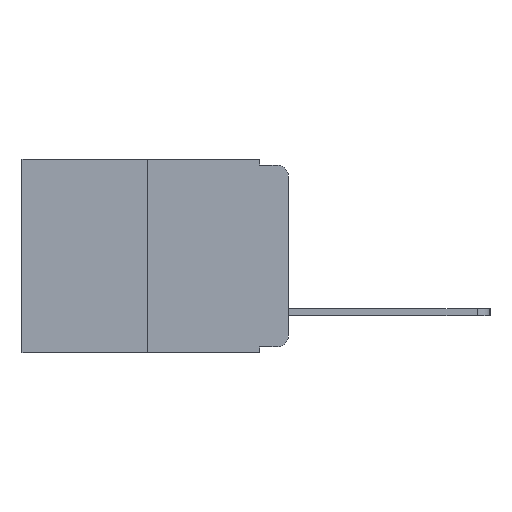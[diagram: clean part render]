
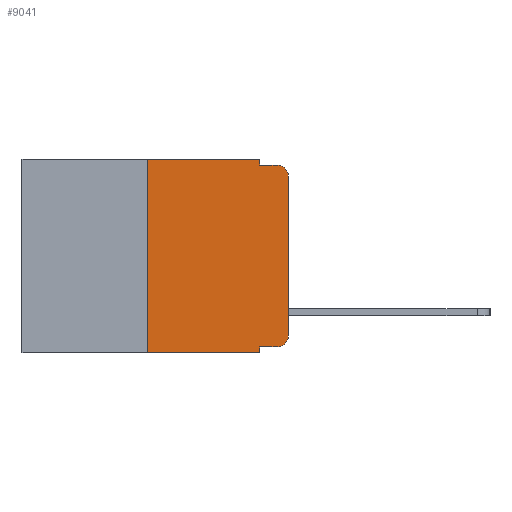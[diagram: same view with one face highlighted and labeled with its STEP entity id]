
A CAD part, left-side view. The second image highlights one B-rep face of the part: STEP entity #9041.
In plain terms, the highlighted planar face has unit normal (-1, 0, 0).
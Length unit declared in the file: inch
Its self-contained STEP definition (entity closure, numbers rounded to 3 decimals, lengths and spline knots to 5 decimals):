
#96 = VERTEX_POINT ( 'NONE', #9918 ) ;
#319 = VECTOR ( 'NONE', #16086, 39.37008 ) ;
#393 = CIRCLE ( 'NONE', #17714, 0.02 ) ;
#594 = CIRCLE ( 'NONE', #8922, 0.02 ) ;
#657 = VECTOR ( 'NONE', #15133, 39.37008 ) ;
#717 = ORIENTED_EDGE ( 'NONE', *, *, #3122, .F. ) ;
#875 = VERTEX_POINT ( 'NONE', #1205 ) ;
#893 = ORIENTED_EDGE ( 'NONE', *, *, #9082, .F. ) ;
#928 = DIRECTION ( 'NONE',  ( 0., 0., -1. ) ) ;
#1081 = DIRECTION ( 'NONE',  ( 0., -1., 0. ) ) ;
#1205 = CARTESIAN_POINT ( 'NONE',  ( 0., 0.25, -0.343 ) ) ;
#1223 = PLANE ( 'NONE',  #4528 ) ;
#1341 = CARTESIAN_POINT ( 'NONE',  ( 0., 0.051, 0. ) ) ;
#1785 = LINE ( 'NONE', #11990, #17336 ) ;
#1945 = EDGE_CURVE ( 'NONE', #14751, #2156, #1785, .T. ) ;
#2156 = VERTEX_POINT ( 'NONE', #3057 ) ;
#2328 = CARTESIAN_POINT ( 'NONE',  ( 0., 0.02, -0.03 ) ) ;
#2532 = DIRECTION ( 'NONE',  ( 0., -1., 0. ) ) ;
#2783 = DIRECTION ( 'NONE',  ( 0., 0., -1. ) ) ;
#2944 = VECTOR ( 'NONE', #19166, 39.37008 ) ;
#3057 = CARTESIAN_POINT ( 'NONE',  ( 0., 0.02, -0.333 ) ) ;
#3122 = EDGE_CURVE ( 'NONE', #875, #96, #18352, .T. ) ;
#3203 = LINE ( 'NONE', #9108, #17700 ) ;
#3656 = ORIENTED_EDGE ( 'NONE', *, *, #14889, .F. ) ;
#3678 = CARTESIAN_POINT ( 'NONE',  ( 0., 0.02, -0.01 ) ) ;
#3746 = ORIENTED_EDGE ( 'NONE', *, *, #10701, .F. ) ;
#3932 = VERTEX_POINT ( 'NONE', #4978 ) ;
#3973 = DIRECTION ( 'NONE',  ( 0., 0., -1. ) ) ;
#4044 = CARTESIAN_POINT ( 'NONE',  ( 0., 0.051, 0. ) ) ;
#4060 = ORIENTED_EDGE ( 'NONE', *, *, #1945, .T. ) ;
#4506 = VERTEX_POINT ( 'NONE', #6914 ) ;
#4528 = AXIS2_PLACEMENT_3D ( 'NONE', #10800, #12207, #2783 ) ;
#4884 = LINE ( 'NONE', #19251, #657 ) ;
#4978 = CARTESIAN_POINT ( 'NONE',  ( 0., 0.051, -0.01 ) ) ;
#5697 = CARTESIAN_POINT ( 'NONE',  ( 0., 0.473, -0.343 ) ) ;
#5799 = ORIENTED_EDGE ( 'NONE', *, *, #13644, .F. ) ;
#5826 = CARTESIAN_POINT ( 'NONE',  ( 0., 0.25, 0. ) ) ;
#6388 = VERTEX_POINT ( 'NONE', #7900 ) ;
#6914 = CARTESIAN_POINT ( 'NONE',  ( 0., 0.051, -0.343 ) ) ;
#7900 = CARTESIAN_POINT ( 'NONE',  ( 0., 0., -0.03 ) ) ;
#8278 = EDGE_CURVE ( 'NONE', #13707, #6388, #9458, .T. ) ;
#8922 = AXIS2_PLACEMENT_3D ( 'NONE', #18866, #10520, #928 ) ;
#9041 = ADVANCED_FACE ( 'NONE', ( #17615 ), #1223, .F. ) ;
#9082 = EDGE_CURVE ( 'NONE', #96, #10858, #4884, .T. ) ;
#9108 = CARTESIAN_POINT ( 'NONE',  ( 0., 0.051, -0.01 ) ) ;
#9346 = DIRECTION ( 'NONE',  ( 0., 0., 1. ) ) ;
#9458 = LINE ( 'NONE', #17753, #16135 ) ;
#9918 = CARTESIAN_POINT ( 'NONE',  ( 0., 0.25, 0. ) ) ;
#10100 = VERTEX_POINT ( 'NONE', #3678 ) ;
#10143 = EDGE_CURVE ( 'NONE', #6388, #10100, #393, .T. ) ;
#10520 = DIRECTION ( 'NONE',  ( -1., 0., 0. ) ) ;
#10536 = LINE ( 'NONE', #4044, #14276 ) ;
#10603 = CARTESIAN_POINT ( 'NONE',  ( 0., 0.051, 0. ) ) ;
#10701 = EDGE_CURVE ( 'NONE', #10858, #3932, #12592, .T. ) ;
#10800 = CARTESIAN_POINT ( 'NONE',  ( 0., 0.473, 0. ) ) ;
#10858 = VERTEX_POINT ( 'NONE', #1341 ) ;
#11268 = EDGE_CURVE ( 'NONE', #2156, #13707, #594, .T. ) ;
#11990 = CARTESIAN_POINT ( 'NONE',  ( 0., 0.051, -0.333 ) ) ;
#12020 = DIRECTION ( 'NONE',  ( 0., 0., -1. ) ) ;
#12207 = DIRECTION ( 'NONE',  ( 1., 0., 0. ) ) ;
#12533 = EDGE_CURVE ( 'NONE', #875, #4506, #16458, .T. ) ;
#12592 = LINE ( 'NONE', #10603, #16710 ) ;
#12933 = ORIENTED_EDGE ( 'NONE', *, *, #10143, .T. ) ;
#13224 = DIRECTION ( 'NONE',  ( -1., 0., 0. ) ) ;
#13285 = DIRECTION ( 'NONE',  ( 0., 0., -1. ) ) ;
#13644 = EDGE_CURVE ( 'NONE', #14751, #4506, #10536, .T. ) ;
#13707 = VERTEX_POINT ( 'NONE', #17509 ) ;
#14276 = VECTOR ( 'NONE', #13285, 39.37008 ) ;
#14751 = VERTEX_POINT ( 'NONE', #17427 ) ;
#14889 = EDGE_CURVE ( 'NONE', #3932, #10100, #3203, .T. ) ;
#15133 = DIRECTION ( 'NONE',  ( 0., -1., 0. ) ) ;
#15547 = EDGE_LOOP ( 'NONE', ( #17823, #12933, #3656, #3746, #893, #717, #19090, #5799, #4060, #19195 ) ) ;
#16086 = DIRECTION ( 'NONE',  ( 0., -1., 0. ) ) ;
#16135 = VECTOR ( 'NONE', #9346, 39.37008 ) ;
#16458 = LINE ( 'NONE', #5697, #319 ) ;
#16710 = VECTOR ( 'NONE', #12020, 39.37008 ) ;
#17336 = VECTOR ( 'NONE', #2532, 39.37008 ) ;
#17427 = CARTESIAN_POINT ( 'NONE',  ( 0., 0.051, -0.333 ) ) ;
#17509 = CARTESIAN_POINT ( 'NONE',  ( 0., 0., -0.313 ) ) ;
#17615 = FACE_OUTER_BOUND ( 'NONE', #15547, .T. ) ;
#17700 = VECTOR ( 'NONE', #1081, 39.37008 ) ;
#17714 = AXIS2_PLACEMENT_3D ( 'NONE', #2328, #13224, #3973 ) ;
#17753 = CARTESIAN_POINT ( 'NONE',  ( 0., 0., 0. ) ) ;
#17823 = ORIENTED_EDGE ( 'NONE', *, *, #8278, .T. ) ;
#18352 = LINE ( 'NONE', #5826, #2944 ) ;
#18866 = CARTESIAN_POINT ( 'NONE',  ( 0., 0.02, -0.313 ) ) ;
#19090 = ORIENTED_EDGE ( 'NONE', *, *, #12533, .T. ) ;
#19166 = DIRECTION ( 'NONE',  ( 0., 0., 1. ) ) ;
#19195 = ORIENTED_EDGE ( 'NONE', *, *, #11268, .T. ) ;
#19251 = CARTESIAN_POINT ( 'NONE',  ( 0., 0.473, 0. ) ) ;
